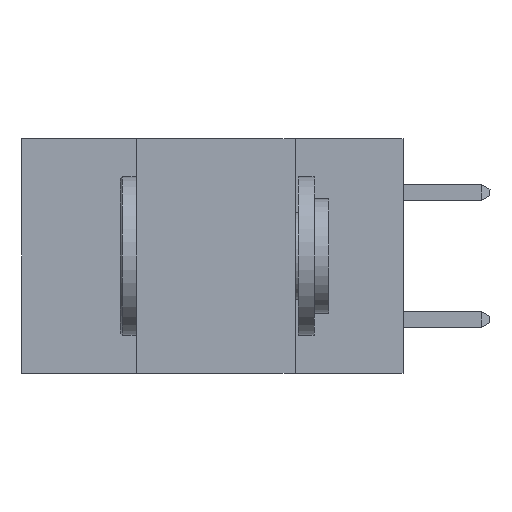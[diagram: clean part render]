
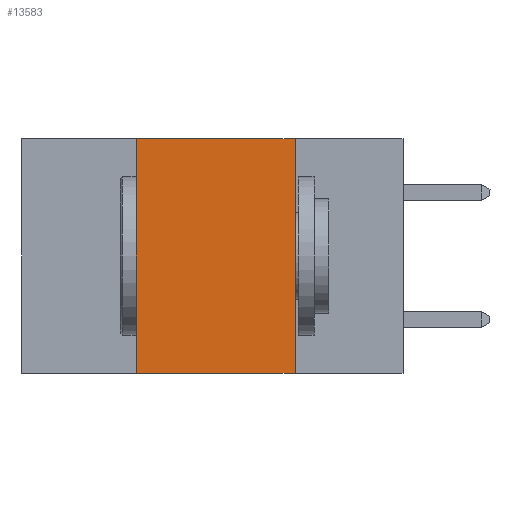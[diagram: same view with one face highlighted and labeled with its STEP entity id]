
A CAD part, left-side view. The second image highlights one B-rep face of the part: STEP entity #13583.
In plain terms, the highlighted planar face has unit normal (-1, 0, 0).
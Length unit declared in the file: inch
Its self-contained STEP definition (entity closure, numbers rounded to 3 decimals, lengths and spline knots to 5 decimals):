
#139 = DIRECTION ( 'NONE',  ( 0., 0., 1. ) ) ;
#289 = LINE ( 'NONE', #2706, #3275 ) ;
#627 = AXIS2_PLACEMENT_3D ( 'NONE', #11067, #5064, #13421 ) ;
#1017 = DIRECTION ( 'NONE',  ( 0., -1., 0. ) ) ;
#1348 = VECTOR ( 'NONE', #2060, 39.37008 ) ;
#2060 = DIRECTION ( 'NONE',  ( 0., 0., -1. ) ) ;
#2646 = PLANE ( 'NONE',  #627 ) ;
#2706 = CARTESIAN_POINT ( 'NONE',  ( 0., 0.42, 0. ) ) ;
#3183 = VECTOR ( 'NONE', #7640, 39.37008 ) ;
#3265 = VERTEX_POINT ( 'NONE', #9594 ) ;
#3272 = VECTOR ( 'NONE', #1017, 39.37008 ) ;
#3275 = VECTOR ( 'NONE', #139, 39.37008 ) ;
#3476 = ORIENTED_EDGE ( 'NONE', *, *, #13662, .F. ) ;
#3626 = VERTEX_POINT ( 'NONE', #5744 ) ;
#3647 = LINE ( 'NONE', #7173, #3272 ) ;
#5064 = DIRECTION ( 'NONE',  ( 1., 0., 0. ) ) ;
#5744 = CARTESIAN_POINT ( 'NONE',  ( 0., 0.42, 0. ) ) ;
#6010 = LINE ( 'NONE', #14668, #3183 ) ;
#6651 = CARTESIAN_POINT ( 'NONE',  ( 0., 0.17, 0. ) ) ;
#7173 = CARTESIAN_POINT ( 'NONE',  ( 0., 0.6, -0.37 ) ) ;
#7640 = DIRECTION ( 'NONE',  ( 0., -1., 0. ) ) ;
#8257 = LINE ( 'NONE', #9312, #1348 ) ;
#9114 = EDGE_CURVE ( 'NONE', #3265, #15239, #3647, .T. ) ;
#9312 = CARTESIAN_POINT ( 'NONE',  ( 0., 0.17, 0. ) ) ;
#9594 = CARTESIAN_POINT ( 'NONE',  ( 0., 0.42, -0.37 ) ) ;
#9902 = EDGE_CURVE ( 'NONE', #3265, #3626, #289, .T. ) ;
#10043 = ORIENTED_EDGE ( 'NONE', *, *, #9902, .F. ) ;
#11067 = CARTESIAN_POINT ( 'NONE',  ( 0., 0.6, 0. ) ) ;
#12321 = ORIENTED_EDGE ( 'NONE', *, *, #15396, .F. ) ;
#12483 = EDGE_LOOP ( 'NONE', ( #12321, #3476, #10043, #13562 ) ) ;
#12651 = CARTESIAN_POINT ( 'NONE',  ( 0., 0.17, -0.37 ) ) ;
#13106 = FACE_OUTER_BOUND ( 'NONE', #12483, .T. ) ;
#13421 = DIRECTION ( 'NONE',  ( 0., 0., -1. ) ) ;
#13562 = ORIENTED_EDGE ( 'NONE', *, *, #9114, .T. ) ;
#13583 = ADVANCED_FACE ( 'NONE', ( #13106 ), #2646, .F. ) ;
#13662 = EDGE_CURVE ( 'NONE', #3626, #15223, #6010, .T. ) ;
#14668 = CARTESIAN_POINT ( 'NONE',  ( 0., 0.6, 0. ) ) ;
#15223 = VERTEX_POINT ( 'NONE', #6651 ) ;
#15239 = VERTEX_POINT ( 'NONE', #12651 ) ;
#15396 = EDGE_CURVE ( 'NONE', #15223, #15239, #8257, .T. ) ;
